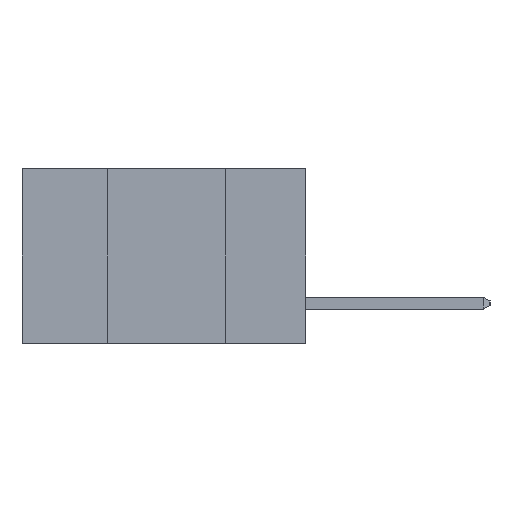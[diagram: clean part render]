
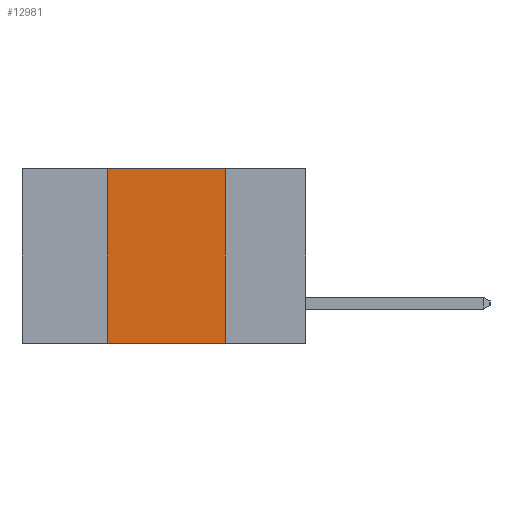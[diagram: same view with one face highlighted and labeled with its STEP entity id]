
A CAD part, left-side view. The second image highlights one B-rep face of the part: STEP entity #12981.
In plain terms, the highlighted planar face has unit normal (-1, 0, 0).
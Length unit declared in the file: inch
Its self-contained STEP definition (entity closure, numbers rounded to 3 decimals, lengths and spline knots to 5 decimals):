
#1481 = CARTESIAN_POINT ( 'NONE',  ( 0., 0.42, 0. ) ) ;
#1892 = VECTOR ( 'NONE', #8938, 39.37008 ) ;
#2143 = PLANE ( 'NONE',  #31781 ) ;
#2726 = ORIENTED_EDGE ( 'NONE', *, *, #15841, .T. ) ;
#4415 = EDGE_LOOP ( 'NONE', ( #5470, #12061, #20183, #2726 ) ) ;
#4519 = VERTEX_POINT ( 'NONE', #10604 ) ;
#5273 = VERTEX_POINT ( 'NONE', #8514 ) ;
#5297 = CARTESIAN_POINT ( 'NONE',  ( 0., 0.42, -0.37 ) ) ;
#5470 = ORIENTED_EDGE ( 'NONE', *, *, #11898, .F. ) ;
#7210 = DIRECTION ( 'NONE',  ( 0., 0., -1. ) ) ;
#7586 = CARTESIAN_POINT ( 'NONE',  ( 0., 0.17, 0. ) ) ;
#8514 = CARTESIAN_POINT ( 'NONE',  ( 0., 0.17, -0.37 ) ) ;
#8938 = DIRECTION ( 'NONE',  ( 0., 0., 1. ) ) ;
#9233 = VERTEX_POINT ( 'NONE', #5297 ) ;
#9407 = DIRECTION ( 'NONE',  ( 0., -1., 0. ) ) ;
#9925 = LINE ( 'NONE', #7586, #19949 ) ;
#10604 = CARTESIAN_POINT ( 'NONE',  ( 0., 0.17, 0. ) ) ;
#10847 = VECTOR ( 'NONE', #19602, 39.37008 ) ;
#11898 = EDGE_CURVE ( 'NONE', #4519, #5273, #9925, .T. ) ;
#12061 = ORIENTED_EDGE ( 'NONE', *, *, #18056, .F. ) ;
#12981 = ADVANCED_FACE ( 'NONE', ( #20257 ), #2143, .F. ) ;
#14737 = VERTEX_POINT ( 'NONE', #15558 ) ;
#15558 = CARTESIAN_POINT ( 'NONE',  ( 0., 0.42, 0. ) ) ;
#15841 = EDGE_CURVE ( 'NONE', #9233, #5273, #17424, .T. ) ;
#17424 = LINE ( 'NONE', #19499, #10847 ) ;
#18056 = EDGE_CURVE ( 'NONE', #14737, #4519, #20713, .T. ) ;
#19499 = CARTESIAN_POINT ( 'NONE',  ( 0., 0.6, -0.37 ) ) ;
#19519 = CARTESIAN_POINT ( 'NONE',  ( 0., 0.6, 0. ) ) ;
#19602 = DIRECTION ( 'NONE',  ( 0., -1., 0. ) ) ;
#19949 = VECTOR ( 'NONE', #29739, 39.37008 ) ;
#20183 = ORIENTED_EDGE ( 'NONE', *, *, #20794, .F. ) ;
#20257 = FACE_OUTER_BOUND ( 'NONE', #4415, .T. ) ;
#20713 = LINE ( 'NONE', #24175, #27210 ) ;
#20794 = EDGE_CURVE ( 'NONE', #9233, #14737, #21675, .T. ) ;
#21675 = LINE ( 'NONE', #1481, #1892 ) ;
#21988 = DIRECTION ( 'NONE',  ( 1., 0., 0. ) ) ;
#24175 = CARTESIAN_POINT ( 'NONE',  ( 0., 0.6, 0. ) ) ;
#27210 = VECTOR ( 'NONE', #9407, 39.37008 ) ;
#29739 = DIRECTION ( 'NONE',  ( 0., 0., -1. ) ) ;
#31781 = AXIS2_PLACEMENT_3D ( 'NONE', #19519, #21988, #7210 ) ;
